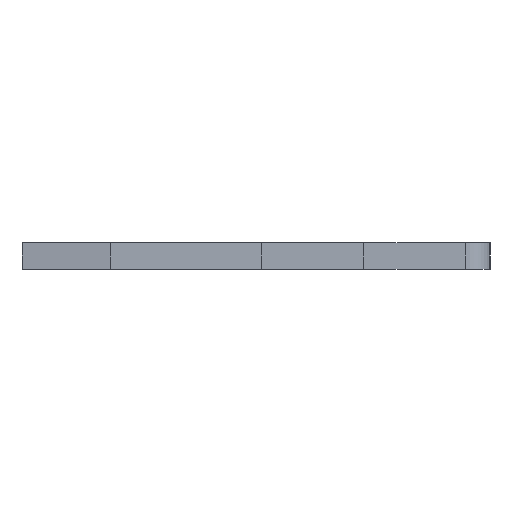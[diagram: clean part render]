
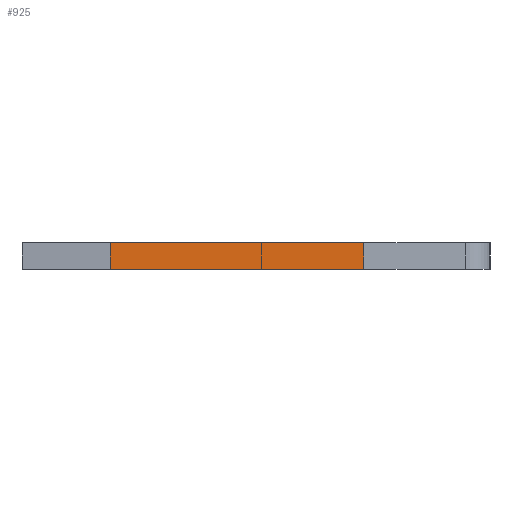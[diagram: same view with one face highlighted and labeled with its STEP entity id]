
A CAD part, left-side view. The second image highlights one B-rep face of the part: STEP entity #925.
In plain terms, the highlighted face is planar.
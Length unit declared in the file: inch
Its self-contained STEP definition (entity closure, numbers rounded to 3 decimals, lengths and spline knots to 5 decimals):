
#64 = DIRECTION ( 'NONE',  ( 0., 1., 0. ) ) ;
#106 = LINE ( 'NONE', #1151, #302 ) ;
#136 = CARTESIAN_POINT ( 'NONE',  ( -0.013, 0.146, -0.0575 ) ) ;
#186 = EDGE_LOOP ( 'NONE', ( #1321, #1834, #1805, #1312 ) ) ;
#249 = EDGE_CURVE ( 'NONE', #2087, #2110, #106, .T. ) ;
#302 = VECTOR ( 'NONE', #1754, 39.37008 ) ;
#310 = CARTESIAN_POINT ( 'NONE',  ( 0.013, 0.146, -0.0575 ) ) ;
#371 = CARTESIAN_POINT ( 'NONE',  ( 0.013, 0.146, -0.0575 ) ) ;
#552 = PLANE ( 'NONE',  #697 ) ;
#643 = CARTESIAN_POINT ( 'NONE',  ( -0.013, 0.146, -0.0575 ) ) ;
#697 = AXIS2_PLACEMENT_3D ( 'NONE', #371, #731, #2176 ) ;
#731 = DIRECTION ( 'NONE',  ( 0., 0., 1. ) ) ;
#788 = DIRECTION ( 'NONE',  ( -1., 0., 0. ) ) ;
#802 = VERTEX_POINT ( 'NONE', #2163 ) ;
#856 = LINE ( 'NONE', #1886, #880 ) ;
#880 = VECTOR ( 'NONE', #788, 39.37008 ) ;
#925 = ADVANCED_FACE ( 'NONE', ( #2032 ), #552, .F. ) ;
#1151 = CARTESIAN_POINT ( 'NONE',  ( 0.013, 0.146, -0.0575 ) ) ;
#1312 = ORIENTED_EDGE ( 'NONE', *, *, #1943, .T. ) ;
#1321 = ORIENTED_EDGE ( 'NONE', *, *, #2128, .T. ) ;
#1585 = DIRECTION ( 'NONE',  ( 0., 1., 0. ) ) ;
#1628 = EDGE_CURVE ( 'NONE', #802, #2087, #2237, .T. ) ;
#1698 = CARTESIAN_POINT ( 'NONE',  ( 0.013, 0.146, -0.0575 ) ) ;
#1754 = DIRECTION ( 'NONE',  ( -1., 0., 0. ) ) ;
#1785 = VECTOR ( 'NONE', #1585, 39.37008 ) ;
#1805 = ORIENTED_EDGE ( 'NONE', *, *, #1628, .F. ) ;
#1834 = ORIENTED_EDGE ( 'NONE', *, *, #249, .F. ) ;
#1886 = CARTESIAN_POINT ( 'NONE',  ( 0.013, -0.099, -0.0575 ) ) ;
#1943 = EDGE_CURVE ( 'NONE', #802, #2166, #856, .T. ) ;
#2032 = FACE_OUTER_BOUND ( 'NONE', #186, .T. ) ;
#2087 = VERTEX_POINT ( 'NONE', #310 ) ;
#2110 = VERTEX_POINT ( 'NONE', #136 ) ;
#2123 = CARTESIAN_POINT ( 'NONE',  ( -0.013, -0.099, -0.0575 ) ) ;
#2128 = EDGE_CURVE ( 'NONE', #2166, #2110, #2263, .T. ) ;
#2135 = VECTOR ( 'NONE', #64, 39.37008 ) ;
#2163 = CARTESIAN_POINT ( 'NONE',  ( 0.013, -0.099, -0.0575 ) ) ;
#2166 = VERTEX_POINT ( 'NONE', #2123 ) ;
#2176 = DIRECTION ( 'NONE',  ( 1., 0., 0. ) ) ;
#2237 = LINE ( 'NONE', #1698, #2135 ) ;
#2263 = LINE ( 'NONE', #643, #1785 ) ;
